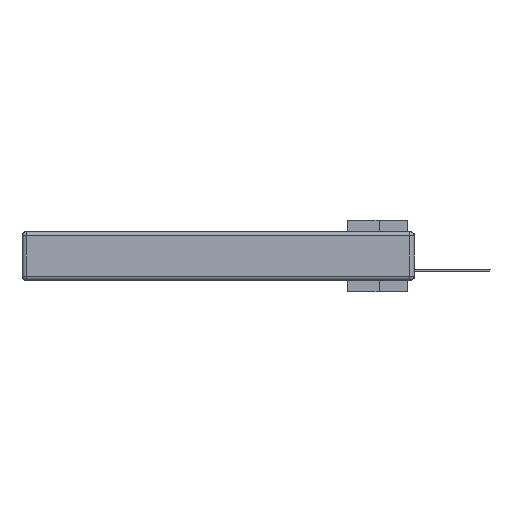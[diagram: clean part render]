
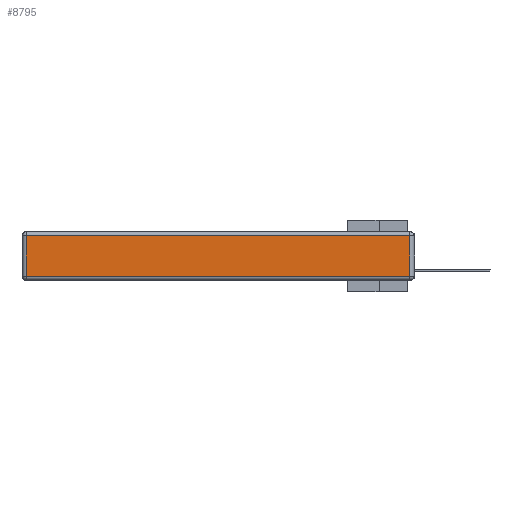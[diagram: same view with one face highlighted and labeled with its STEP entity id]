
A CAD part, left-side view. The second image highlights one B-rep face of the part: STEP entity #8795.
In plain terms, the highlighted planar face has unit normal (-1, 0, 0).
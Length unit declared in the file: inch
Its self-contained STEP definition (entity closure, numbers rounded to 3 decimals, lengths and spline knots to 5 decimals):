
#257 = VERTEX_POINT ( 'NONE', #4286 ) ;
#1696 = CARTESIAN_POINT ( 'NONE',  ( 0., 2.72, -0.03 ) ) ;
#2399 = ORIENTED_EDGE ( 'NONE', *, *, #9738, .T. ) ;
#2928 = LINE ( 'NONE', #8084, #16616 ) ;
#4205 = ORIENTED_EDGE ( 'NONE', *, *, #9033, .T. ) ;
#4286 = CARTESIAN_POINT ( 'NONE',  ( 0., 2.72, -0.313 ) ) ;
#5496 = DIRECTION ( 'NONE',  ( 0., 1., 0. ) ) ;
#5792 = CARTESIAN_POINT ( 'NONE',  ( 0., 0., -0.313 ) ) ;
#7026 = FACE_OUTER_BOUND ( 'NONE', #10890, .T. ) ;
#8084 = CARTESIAN_POINT ( 'NONE',  ( 0., 2.75, -0.03 ) ) ;
#8374 = VERTEX_POINT ( 'NONE', #14064 ) ;
#8795 = ADVANCED_FACE ( 'NONE', ( #7026 ), #10064, .T. ) ;
#9033 = EDGE_CURVE ( 'NONE', #29802, #8374, #14043, .T. ) ;
#9419 = EDGE_CURVE ( 'NONE', #14863, #257, #10317, .T. ) ;
#9738 = EDGE_CURVE ( 'NONE', #257, #29802, #20347, .T. ) ;
#10064 = PLANE ( 'NONE',  #17344 ) ;
#10317 = LINE ( 'NONE', #19044, #23310 ) ;
#10890 = EDGE_LOOP ( 'NONE', ( #2399, #4205, #29906, #22326 ) ) ;
#13449 = CARTESIAN_POINT ( 'NONE',  ( 0., 0.03, -0.313 ) ) ;
#14043 = LINE ( 'NONE', #15006, #21472 ) ;
#14064 = CARTESIAN_POINT ( 'NONE',  ( 0., 0.03, -0.03 ) ) ;
#14863 = VERTEX_POINT ( 'NONE', #1696 ) ;
#15006 = CARTESIAN_POINT ( 'NONE',  ( 0., 0.03, -0.343 ) ) ;
#15045 = DIRECTION ( 'NONE',  ( -1., 0., 0. ) ) ;
#16616 = VECTOR ( 'NONE', #5496, 39.37008 ) ;
#17344 = AXIS2_PLACEMENT_3D ( 'NONE', #19718, #15045, #22006 ) ;
#19044 = CARTESIAN_POINT ( 'NONE',  ( 0., 2.72, -0.343 ) ) ;
#19145 = DIRECTION ( 'NONE',  ( 0., 0., -1. ) ) ;
#19718 = CARTESIAN_POINT ( 'NONE',  ( 0., 0., -0.343 ) ) ;
#20347 = LINE ( 'NONE', #5792, #26973 ) ;
#21472 = VECTOR ( 'NONE', #24441, 39.37008 ) ;
#22006 = DIRECTION ( 'NONE',  ( 0., 0., 1. ) ) ;
#22326 = ORIENTED_EDGE ( 'NONE', *, *, #9419, .T. ) ;
#23310 = VECTOR ( 'NONE', #19145, 39.37008 ) ;
#24441 = DIRECTION ( 'NONE',  ( 0., 0., 1. ) ) ;
#26973 = VECTOR ( 'NONE', #27128, 39.37008 ) ;
#27128 = DIRECTION ( 'NONE',  ( 0., -1., 0. ) ) ;
#28614 = EDGE_CURVE ( 'NONE', #8374, #14863, #2928, .T. ) ;
#29802 = VERTEX_POINT ( 'NONE', #13449 ) ;
#29906 = ORIENTED_EDGE ( 'NONE', *, *, #28614, .T. ) ;
